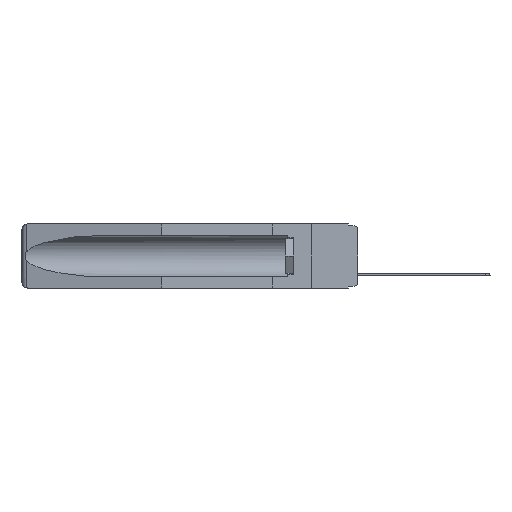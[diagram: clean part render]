
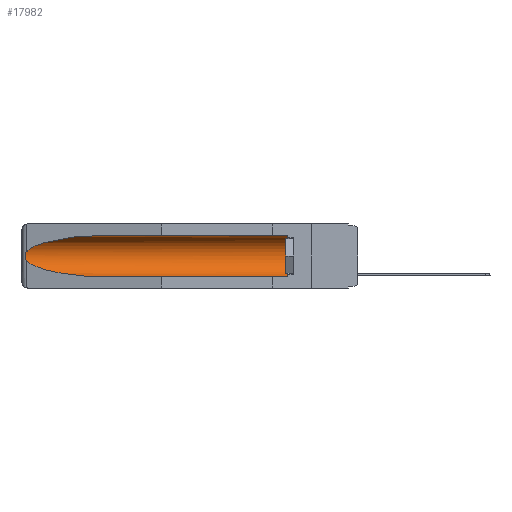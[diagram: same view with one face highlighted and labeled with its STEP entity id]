
A CAD part, left-side view. The second image highlights one B-rep face of the part: STEP entity #17982.
In plain terms, the highlighted cylindrical face has radius 2.857 mm (diameter 5.715 mm), a partial arc.
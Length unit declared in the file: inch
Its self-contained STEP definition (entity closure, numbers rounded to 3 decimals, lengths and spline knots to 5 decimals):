
#108 = DIRECTION ( 'NONE',  ( 0., 0., 1. ) ) ;
#736 = CYLINDRICAL_SURFACE ( 'NONE', #6294, 0.1125 ) ;
#737 = ORIENTED_EDGE ( 'NONE', *, *, #3325, .T. ) ;
#810 = EDGE_CURVE ( 'NONE', #16267, #18309, #16002, .T. ) ;
#941 = CARTESIAN_POINT ( 'NONE',  ( 0.26597, 1.5296, -0.19026 ) ) ;
#1025 =( BOUNDED_CURVE ( )  B_SPLINE_CURVE ( 3, ( #10162, #14577, #8827, #11559 ),
 .UNSPECIFIED., .F., .F. ) 
 B_SPLINE_CURVE_WITH_KNOTS ( ( 4, 4 ),
 ( 0.1948, 1.5708 ),
 .UNSPECIFIED. ) 
 CURVE ( )  GEOMETRIC_REPRESENTATION_ITEM ( )  RATIONAL_B_SPLINE_CURVE ( ( 1., 0.848, 0.848, 1. ) ) 
 REPRESENTATION_ITEM ( '' )  );
#1174 = DIRECTION ( 'NONE',  ( 0., 1., 0. ) ) ;
#1771 = CARTESIAN_POINT ( 'NONE',  ( 0.155, -0.30754, -0.284 ) ) ;
#1962 = CARTESIAN_POINT ( 'NONE',  ( 0.25451, 1.48313, -0.09465 ) ) ;
#2050 = B_SPLINE_CURVE_WITH_KNOTS ( 'NONE', 3,
 ( #10396, #8093, #12829, #10566, #9531, #12567, #15336, #5315, #941, #18266 ),
 .UNSPECIFIED., .F., .F.,
 ( 4, 2, 2, 2, 4 ),
 ( 0., 0.00029, 0.00058, 0.00087, 0.00117 ),
 .UNSPECIFIED. ) ;
#3325 = EDGE_CURVE ( 'NONE', #18334, #4755, #1025, .T. ) ;
#3657 = CARTESIAN_POINT ( 'NONE',  ( 0.155, 1.07973, -0.059 ) ) ;
#4053 = CARTESIAN_POINT ( 'NONE',  ( 0.155, -0.30754, -0.059 ) ) ;
#4614 = EDGE_CURVE ( 'NONE', #15603, #4755, #12529, .T. ) ;
#4705 = ORIENTED_EDGE ( 'NONE', *, *, #11297, .T. ) ;
#4755 = VERTEX_POINT ( 'NONE', #15211 ) ;
#5315 = CARTESIAN_POINT ( 'NONE',  ( 0.26655, 1.53094, -0.18657 ) ) ;
#5567 = CARTESIAN_POINT ( 'NONE',  ( 0.155, 0.126, -0.284 ) ) ;
#5657 = DIRECTION ( 'NONE',  ( 0., 1., 0. ) ) ;
#5757 = CARTESIAN_POINT ( 'NONE',  ( 0.155, 1.07973, -0.059 ) ) ;
#6048 = ORIENTED_EDGE ( 'NONE', *, *, #810, .T. ) ;
#6294 = AXIS2_PLACEMENT_3D ( 'NONE', #7045, #5657, #9753 ) ;
#7045 = CARTESIAN_POINT ( 'NONE',  ( 0.155, -0.30754, -0.1715 ) ) ;
#7128 = CIRCLE ( 'NONE', #16899, 0.1125 ) ;
#7580 = ORIENTED_EDGE ( 'NONE', *, *, #4614, .F. ) ;
#7818 = CARTESIAN_POINT ( 'NONE',  ( 0.21114, 1.30732, -0.059 ) ) ;
#7947 = CARTESIAN_POINT ( 'NONE',  ( 0.26537, 1.52718, -0.14972 ) ) ;
#7985 = CARTESIAN_POINT ( 'NONE',  ( 0.26537, 1.52718, -0.19328 ) ) ;
#8093 = CARTESIAN_POINT ( 'NONE',  ( 0.26597, 1.52961, -0.15275 ) ) ;
#8296 = VECTOR ( 'NONE', #1174, 39.37008 ) ;
#8827 = CARTESIAN_POINT ( 'NONE',  ( 0.21114, 1.30732, -0.284 ) ) ;
#8899 = ORIENTED_EDGE ( 'NONE', *, *, #15644, .T. ) ;
#9531 = CARTESIAN_POINT ( 'NONE',  ( 0.2675, 1.53308, -0.16763 ) ) ;
#9753 = DIRECTION ( 'NONE',  ( 0., 0., 1. ) ) ;
#10162 = CARTESIAN_POINT ( 'NONE',  ( 0.26537, 1.52718, -0.19328 ) ) ;
#10396 = CARTESIAN_POINT ( 'NONE',  ( 0.26537, 1.52718, -0.14972 ) ) ;
#10419 = CARTESIAN_POINT ( 'NONE',  ( 0.155, 0.126, -0.1715 ) ) ;
#10566 = CARTESIAN_POINT ( 'NONE',  ( 0.2673, 1.5327, -0.16383 ) ) ;
#10785 = CARTESIAN_POINT ( 'NONE',  ( 0.155, 0.126, -0.059 ) ) ;
#10836 = CARTESIAN_POINT ( 'NONE',  ( 0.26537, 1.52718, -0.14972 ) ) ;
#11297 = EDGE_CURVE ( 'NONE', #18309, #18334, #2050, .T. ) ;
#11559 = CARTESIAN_POINT ( 'NONE',  ( 0.155, 1.07973, -0.284 ) ) ;
#11871 = EDGE_CURVE ( 'NONE', #12369, #16267, #12118, .T. ) ;
#12118 = LINE ( 'NONE', #4053, #8296 ) ;
#12369 = VERTEX_POINT ( 'NONE', #10785 ) ;
#12529 = LINE ( 'NONE', #1771, #17677 ) ;
#12567 = CARTESIAN_POINT ( 'NONE',  ( 0.2675, 1.53308, -0.17534 ) ) ;
#12829 = CARTESIAN_POINT ( 'NONE',  ( 0.26654, 1.53092, -0.15636 ) ) ;
#14577 = CARTESIAN_POINT ( 'NONE',  ( 0.25451, 1.48313, -0.24835 ) ) ;
#15171 = EDGE_LOOP ( 'NONE', ( #6048, #4705, #737, #7580, #8899, #18207 ) ) ;
#15211 = CARTESIAN_POINT ( 'NONE',  ( 0.155, 1.07973, -0.284 ) ) ;
#15336 = CARTESIAN_POINT ( 'NONE',  ( 0.2673, 1.53269, -0.17917 ) ) ;
#15603 = VERTEX_POINT ( 'NONE', #5567 ) ;
#15644 = EDGE_CURVE ( 'NONE', #15603, #12369, #7128, .T. ) ;
#16002 =( BOUNDED_CURVE ( )  B_SPLINE_CURVE ( 3, ( #3657, #7818, #1962, #7947 ),
 .UNSPECIFIED., .F., .F. ) 
 B_SPLINE_CURVE_WITH_KNOTS ( ( 4, 4 ),
 ( 4.71239, 6.08839 ),
 .UNSPECIFIED. ) 
 CURVE ( )  GEOMETRIC_REPRESENTATION_ITEM ( )  RATIONAL_B_SPLINE_CURVE ( ( 1., 0.848, 0.848, 1. ) ) 
 REPRESENTATION_ITEM ( '' )  );
#16012 = DIRECTION ( 'NONE',  ( 0., -1., 0. ) ) ;
#16122 = DIRECTION ( 'NONE',  ( 0., 1., 0. ) ) ;
#16267 = VERTEX_POINT ( 'NONE', #5757 ) ;
#16708 = FACE_OUTER_BOUND ( 'NONE', #15171, .T. ) ;
#16899 = AXIS2_PLACEMENT_3D ( 'NONE', #10419, #16012, #108 ) ;
#17677 = VECTOR ( 'NONE', #16122, 39.37008 ) ;
#17982 = ADVANCED_FACE ( 'NONE', ( #16708 ), #736, .F. ) ;
#18207 = ORIENTED_EDGE ( 'NONE', *, *, #11871, .T. ) ;
#18266 = CARTESIAN_POINT ( 'NONE',  ( 0.26537, 1.52718, -0.19328 ) ) ;
#18309 = VERTEX_POINT ( 'NONE', #10836 ) ;
#18334 = VERTEX_POINT ( 'NONE', #7985 ) ;
